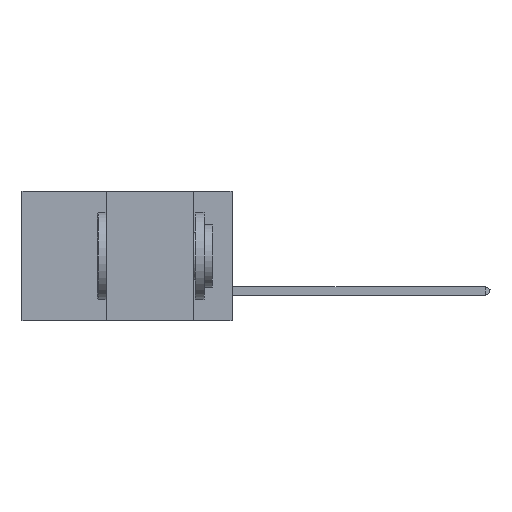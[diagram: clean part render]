
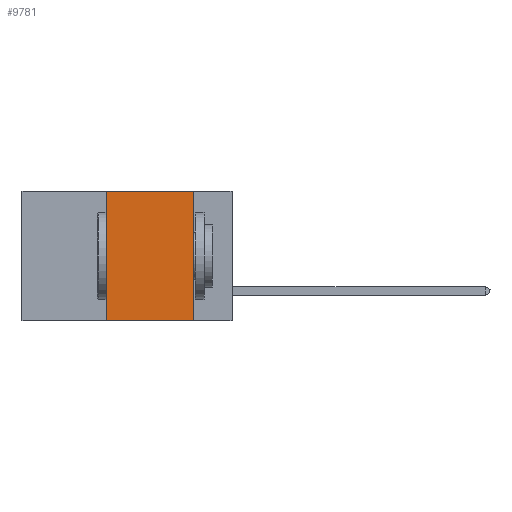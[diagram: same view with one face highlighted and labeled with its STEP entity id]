
A CAD part, left-side view. The second image highlights one B-rep face of the part: STEP entity #9781.
In plain terms, the highlighted planar face has unit normal (-1, 0, 0).
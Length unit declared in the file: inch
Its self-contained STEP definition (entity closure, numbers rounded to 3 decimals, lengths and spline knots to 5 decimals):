
#3140 = CARTESIAN_POINT ( 'NONE',  ( 0., 0.6, -0.37 ) ) ;
#3151 = EDGE_LOOP ( 'NONE', ( #25395, #14783, #10796, #16014 ) ) ;
#3491 = DIRECTION ( 'NONE',  ( 0., 0., -1. ) ) ;
#3518 = LINE ( 'NONE', #12536, #7697 ) ;
#4263 = DIRECTION ( 'NONE',  ( 0., 0., -1. ) ) ;
#4292 = VERTEX_POINT ( 'NONE', #6194 ) ;
#6194 = CARTESIAN_POINT ( 'NONE',  ( 0., 0.36, -0.37 ) ) ;
#6468 = DIRECTION ( 'NONE',  ( 0., -1., 0. ) ) ;
#7261 = VECTOR ( 'NONE', #3491, 39.37008 ) ;
#7390 = AXIS2_PLACEMENT_3D ( 'NONE', #18135, #12445, #4263 ) ;
#7697 = VECTOR ( 'NONE', #24753, 39.37008 ) ;
#7707 = CARTESIAN_POINT ( 'NONE',  ( 0., 0.11, 0. ) ) ;
#7797 = PLANE ( 'NONE',  #7390 ) ;
#7836 = FACE_OUTER_BOUND ( 'NONE', #3151, .T. ) ;
#9171 = LINE ( 'NONE', #3140, #17874 ) ;
#9733 = VERTEX_POINT ( 'NONE', #22096 ) ;
#9781 = ADVANCED_FACE ( 'NONE', ( #7836 ), #7797, .F. ) ;
#10054 = LINE ( 'NONE', #20614, #22898 ) ;
#10127 = EDGE_CURVE ( 'NONE', #12413, #9733, #10054, .T. ) ;
#10796 = ORIENTED_EDGE ( 'NONE', *, *, #24709, .F. ) ;
#12376 = LINE ( 'NONE', #7707, #7261 ) ;
#12413 = VERTEX_POINT ( 'NONE', #20972 ) ;
#12435 = VERTEX_POINT ( 'NONE', #14245 ) ;
#12445 = DIRECTION ( 'NONE',  ( 1., 0., 0. ) ) ;
#12536 = CARTESIAN_POINT ( 'NONE',  ( 0., 0.36, 0. ) ) ;
#14245 = CARTESIAN_POINT ( 'NONE',  ( 0., 0.11, -0.37 ) ) ;
#14783 = ORIENTED_EDGE ( 'NONE', *, *, #10127, .F. ) ;
#15418 = DIRECTION ( 'NONE',  ( 0., -1., 0. ) ) ;
#16014 = ORIENTED_EDGE ( 'NONE', *, *, #22754, .T. ) ;
#17874 = VECTOR ( 'NONE', #15418, 39.37008 ) ;
#18135 = CARTESIAN_POINT ( 'NONE',  ( 0., 0.6, 0. ) ) ;
#20614 = CARTESIAN_POINT ( 'NONE',  ( 0., 0.6, 0. ) ) ;
#20972 = CARTESIAN_POINT ( 'NONE',  ( 0., 0.36, 0. ) ) ;
#22096 = CARTESIAN_POINT ( 'NONE',  ( 0., 0.11, 0. ) ) ;
#22754 = EDGE_CURVE ( 'NONE', #4292, #12435, #9171, .T. ) ;
#22898 = VECTOR ( 'NONE', #6468, 39.37008 ) ;
#22899 = EDGE_CURVE ( 'NONE', #9733, #12435, #12376, .T. ) ;
#24709 = EDGE_CURVE ( 'NONE', #4292, #12413, #3518, .T. ) ;
#24753 = DIRECTION ( 'NONE',  ( 0., 0., 1. ) ) ;
#25395 = ORIENTED_EDGE ( 'NONE', *, *, #22899, .F. ) ;
